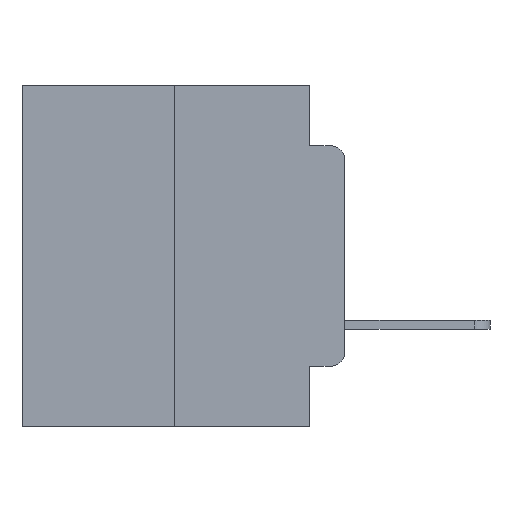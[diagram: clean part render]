
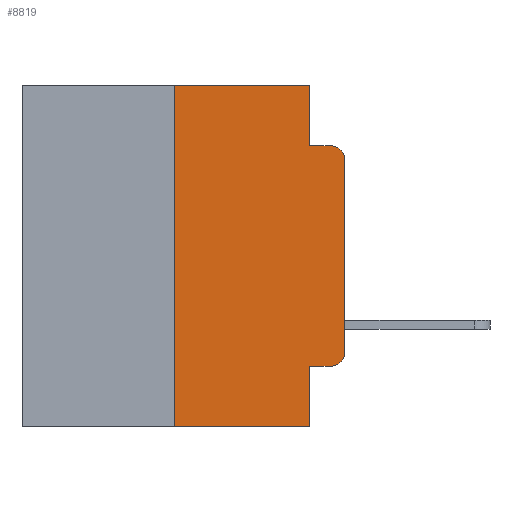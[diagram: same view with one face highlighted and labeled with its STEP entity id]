
A CAD part, left-side view. The second image highlights one B-rep face of the part: STEP entity #8819.
In plain terms, the highlighted planar face has unit normal (-1, 0, 0).
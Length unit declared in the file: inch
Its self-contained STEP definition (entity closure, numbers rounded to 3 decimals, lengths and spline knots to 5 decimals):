
#244 = CARTESIAN_POINT ( 'NONE',  ( 0., 0.25, 0. ) ) ;
#316 = DIRECTION ( 'NONE',  ( 0., 0., 1. ) ) ;
#809 = CARTESIAN_POINT ( 'NONE',  ( 0., 0., 0. ) ) ;
#901 = ORIENTED_EDGE ( 'NONE', *, *, #3470, .T. ) ;
#1098 = CARTESIAN_POINT ( 'NONE',  ( 0., 0.25, 0. ) ) ;
#1882 = VECTOR ( 'NONE', #8484, 39.37008 ) ;
#2182 = VERTEX_POINT ( 'NONE', #16142 ) ;
#2307 = ORIENTED_EDGE ( 'NONE', *, *, #3873, .F. ) ;
#2373 = VERTEX_POINT ( 'NONE', #18241 ) ;
#2540 = DIRECTION ( 'NONE',  ( -1., 0., 0. ) ) ;
#2791 = CARTESIAN_POINT ( 'NONE',  ( 0., 0.02, -0.0885 ) ) ;
#3248 = CARTESIAN_POINT ( 'NONE',  ( 0., 0.051, 0. ) ) ;
#3342 = VERTEX_POINT ( 'NONE', #22024 ) ;
#3465 = EDGE_CURVE ( 'NONE', #16704, #10252, #11101, .T. ) ;
#3470 = EDGE_CURVE ( 'NONE', #10252, #18308, #21483, .T. ) ;
#3519 = EDGE_CURVE ( 'NONE', #2373, #18308, #14468, .T. ) ;
#3692 = ORIENTED_EDGE ( 'NONE', *, *, #22814, .F. ) ;
#3752 = CARTESIAN_POINT ( 'NONE',  ( 0., 0.473, 0. ) ) ;
#3873 = EDGE_CURVE ( 'NONE', #8175, #2373, #20299, .T. ) ;
#3937 = EDGE_CURVE ( 'NONE', #3342, #19563, #19136, .T. ) ;
#3975 = EDGE_CURVE ( 'NONE', #22008, #8246, #26349, .T. ) ;
#3982 = EDGE_CURVE ( 'NONE', #22008, #2182, #25113, .T. ) ;
#4030 = EDGE_CURVE ( 'NONE', #2182, #16704, #8956, .T. ) ;
#5122 = ORIENTED_EDGE ( 'NONE', *, *, #8074, .T. ) ;
#5850 = CARTESIAN_POINT ( 'NONE',  ( 0., 0.051, -0.5 ) ) ;
#6050 = DIRECTION ( 'NONE',  ( 1., 0., 0. ) ) ;
#6751 = CARTESIAN_POINT ( 'NONE',  ( 0., 0.051, -0.4115 ) ) ;
#7238 = VECTOR ( 'NONE', #316, 39.37008 ) ;
#8074 = EDGE_CURVE ( 'NONE', #3342, #8246, #9051, .T. ) ;
#8175 = VERTEX_POINT ( 'NONE', #3248 ) ;
#8246 = VERTEX_POINT ( 'NONE', #5850 ) ;
#8272 = CARTESIAN_POINT ( 'NONE',  ( 0., 0.02, -0.1085 ) ) ;
#8382 = VECTOR ( 'NONE', #9318, 39.37008 ) ;
#8484 = DIRECTION ( 'NONE',  ( 0., -1., 0. ) ) ;
#8819 = ADVANCED_FACE ( 'NONE', ( #23272 ), #16207, .F. ) ;
#8956 = CIRCLE ( 'NONE', #14416, 0.02 ) ;
#9006 = DIRECTION ( 'NONE',  ( 0., 0., 1. ) ) ;
#9051 = LINE ( 'NONE', #11219, #8382 ) ;
#9084 = DIRECTION ( 'NONE',  ( -1., 0., 0. ) ) ;
#9318 = DIRECTION ( 'NONE',  ( 0., -1., 0. ) ) ;
#10252 = VERTEX_POINT ( 'NONE', #11909 ) ;
#10553 = CARTESIAN_POINT ( 'NONE',  ( 0., 0.473, 0. ) ) ;
#10848 = DIRECTION ( 'NONE',  ( 0., 0., -1. ) ) ;
#11101 = LINE ( 'NONE', #809, #25985 ) ;
#11219 = CARTESIAN_POINT ( 'NONE',  ( 0., 0.473, -0.5 ) ) ;
#11644 = CARTESIAN_POINT ( 'NONE',  ( 0., 0.051, -0.0885 ) ) ;
#11689 = DIRECTION ( 'NONE',  ( 0., -1., 0. ) ) ;
#11764 = ORIENTED_EDGE ( 'NONE', *, *, #3465, .T. ) ;
#11909 = CARTESIAN_POINT ( 'NONE',  ( 0., 0., -0.1085 ) ) ;
#11947 = AXIS2_PLACEMENT_3D ( 'NONE', #8272, #2540, #15765 ) ;
#12077 = ORIENTED_EDGE ( 'NONE', *, *, #3982, .T. ) ;
#12371 = ORIENTED_EDGE ( 'NONE', *, *, #3519, .F. ) ;
#12999 = DIRECTION ( 'NONE',  ( 0., 0., -1. ) ) ;
#13211 = LINE ( 'NONE', #10553, #1882 ) ;
#13835 = CARTESIAN_POINT ( 'NONE',  ( 0., 0.051, -0.4115 ) ) ;
#14416 = AXIS2_PLACEMENT_3D ( 'NONE', #20758, #9084, #22724 ) ;
#14468 = LINE ( 'NONE', #11644, #19679 ) ;
#15510 = AXIS2_PLACEMENT_3D ( 'NONE', #3752, #6050, #20078 ) ;
#15765 = DIRECTION ( 'NONE',  ( 0., 0., -1. ) ) ;
#16078 = VECTOR ( 'NONE', #10848, 39.37008 ) ;
#16142 = CARTESIAN_POINT ( 'NONE',  ( 0., 0.02, -0.4115 ) ) ;
#16207 = PLANE ( 'NONE',  #15510 ) ;
#16704 = VERTEX_POINT ( 'NONE', #21093 ) ;
#18241 = CARTESIAN_POINT ( 'NONE',  ( 0., 0.051, -0.0885 ) ) ;
#18308 = VERTEX_POINT ( 'NONE', #2791 ) ;
#18639 = CARTESIAN_POINT ( 'NONE',  ( 0., 0.051, 0. ) ) ;
#19136 = LINE ( 'NONE', #1098, #7238 ) ;
#19563 = VERTEX_POINT ( 'NONE', #244 ) ;
#19679 = VECTOR ( 'NONE', #11689, 39.37008 ) ;
#19742 = VECTOR ( 'NONE', #12999, 39.37008 ) ;
#20000 = VECTOR ( 'NONE', #20681, 39.37008 ) ;
#20078 = DIRECTION ( 'NONE',  ( 0., 0., -1. ) ) ;
#20299 = LINE ( 'NONE', #26014, #19742 ) ;
#20681 = DIRECTION ( 'NONE',  ( 0., -1., 0. ) ) ;
#20758 = CARTESIAN_POINT ( 'NONE',  ( 0., 0.02, -0.3915 ) ) ;
#21093 = CARTESIAN_POINT ( 'NONE',  ( 0., 0., -0.3915 ) ) ;
#21216 = ORIENTED_EDGE ( 'NONE', *, *, #3975, .F. ) ;
#21483 = CIRCLE ( 'NONE', #11947, 0.02 ) ;
#22008 = VERTEX_POINT ( 'NONE', #13835 ) ;
#22024 = CARTESIAN_POINT ( 'NONE',  ( 0., 0.25, -0.5 ) ) ;
#22424 = ORIENTED_EDGE ( 'NONE', *, *, #4030, .T. ) ;
#22724 = DIRECTION ( 'NONE',  ( 0., 0., -1. ) ) ;
#22814 = EDGE_CURVE ( 'NONE', #19563, #8175, #13211, .T. ) ;
#23272 = FACE_OUTER_BOUND ( 'NONE', #24211, .T. ) ;
#24211 = EDGE_LOOP ( 'NONE', ( #11764, #901, #12371, #2307, #3692, #25111, #5122, #21216, #12077, #22424 ) ) ;
#25111 = ORIENTED_EDGE ( 'NONE', *, *, #3937, .F. ) ;
#25113 = LINE ( 'NONE', #6751, #20000 ) ;
#25985 = VECTOR ( 'NONE', #9006, 39.37008 ) ;
#26014 = CARTESIAN_POINT ( 'NONE',  ( 0., 0.051, 0. ) ) ;
#26349 = LINE ( 'NONE', #18639, #16078 ) ;
